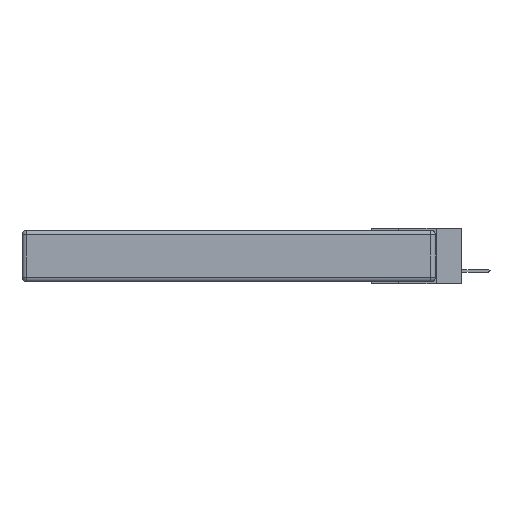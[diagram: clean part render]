
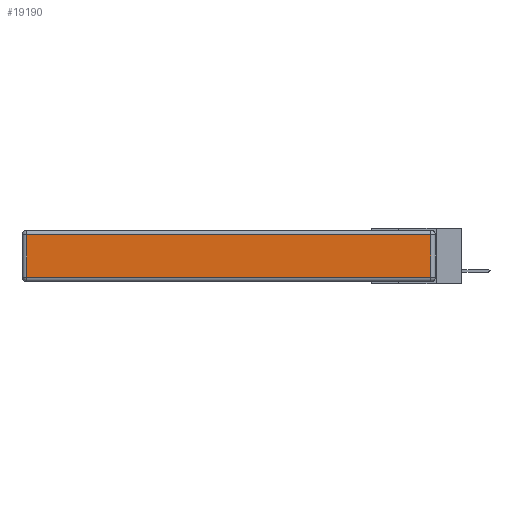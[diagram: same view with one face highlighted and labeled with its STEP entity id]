
A CAD part, left-side view. The second image highlights one B-rep face of the part: STEP entity #19190.
In plain terms, the highlighted planar face has unit normal (-1, 0, 0).
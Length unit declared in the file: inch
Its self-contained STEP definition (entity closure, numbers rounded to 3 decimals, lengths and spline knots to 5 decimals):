
#548 = ORIENTED_EDGE ( 'NONE', *, *, #19795, .T. ) ;
#662 = VERTEX_POINT ( 'NONE', #15623 ) ;
#825 = LINE ( 'NONE', #8303, #12501 ) ;
#1644 = CARTESIAN_POINT ( 'NONE',  ( 0., 0., -0.343 ) ) ;
#3388 = DIRECTION ( 'NONE',  ( 0., -1., 0. ) ) ;
#5921 = DIRECTION ( 'NONE',  ( 0., 0., 1. ) ) ;
#8303 = CARTESIAN_POINT ( 'NONE',  ( 0., 0.03, -0.343 ) ) ;
#8431 = EDGE_LOOP ( 'NONE', ( #14127, #548, #25005, #13392 ) ) ;
#9289 = DIRECTION ( 'NONE',  ( 0., 1., 0. ) ) ;
#9433 = EDGE_CURVE ( 'NONE', #28408, #22156, #24236, .T. ) ;
#9835 = DIRECTION ( 'NONE',  ( 0., 0., -1. ) ) ;
#10641 = VECTOR ( 'NONE', #9289, 39.37008 ) ;
#10645 = EDGE_CURVE ( 'NONE', #15297, #28408, #12044, .T. ) ;
#10659 = DIRECTION ( 'NONE',  ( -1., 0., 0. ) ) ;
#11050 = VECTOR ( 'NONE', #9835, 39.37008 ) ;
#11377 = AXIS2_PLACEMENT_3D ( 'NONE', #1644, #10659, #26256 ) ;
#12044 = LINE ( 'NONE', #22161, #10641 ) ;
#12188 = FACE_OUTER_BOUND ( 'NONE', #8431, .T. ) ;
#12501 = VECTOR ( 'NONE', #5921, 39.37008 ) ;
#13392 = ORIENTED_EDGE ( 'NONE', *, *, #9433, .T. ) ;
#14127 = ORIENTED_EDGE ( 'NONE', *, *, #26784, .T. ) ;
#14692 = CARTESIAN_POINT ( 'NONE',  ( 0., 0., -0.313 ) ) ;
#15297 = VERTEX_POINT ( 'NONE', #28000 ) ;
#15623 = CARTESIAN_POINT ( 'NONE',  ( 0., 0.03, -0.313 ) ) ;
#16742 = CARTESIAN_POINT ( 'NONE',  ( 0., 2.72, -0.343 ) ) ;
#18337 = CARTESIAN_POINT ( 'NONE',  ( 0., 2.72, -0.03 ) ) ;
#19190 = ADVANCED_FACE ( 'NONE', ( #12188 ), #26653, .T. ) ;
#19427 = CARTESIAN_POINT ( 'NONE',  ( 0., 2.72, -0.313 ) ) ;
#19795 = EDGE_CURVE ( 'NONE', #662, #15297, #825, .T. ) ;
#22156 = VERTEX_POINT ( 'NONE', #19427 ) ;
#22161 = CARTESIAN_POINT ( 'NONE',  ( 0., 2.75, -0.03 ) ) ;
#24236 = LINE ( 'NONE', #16742, #11050 ) ;
#25005 = ORIENTED_EDGE ( 'NONE', *, *, #10645, .T. ) ;
#25276 = VECTOR ( 'NONE', #3388, 39.37008 ) ;
#25634 = LINE ( 'NONE', #14692, #25276 ) ;
#26256 = DIRECTION ( 'NONE',  ( 0., 0., 1. ) ) ;
#26653 = PLANE ( 'NONE',  #11377 ) ;
#26784 = EDGE_CURVE ( 'NONE', #22156, #662, #25634, .T. ) ;
#28000 = CARTESIAN_POINT ( 'NONE',  ( 0., 0.03, -0.03 ) ) ;
#28408 = VERTEX_POINT ( 'NONE', #18337 ) ;
